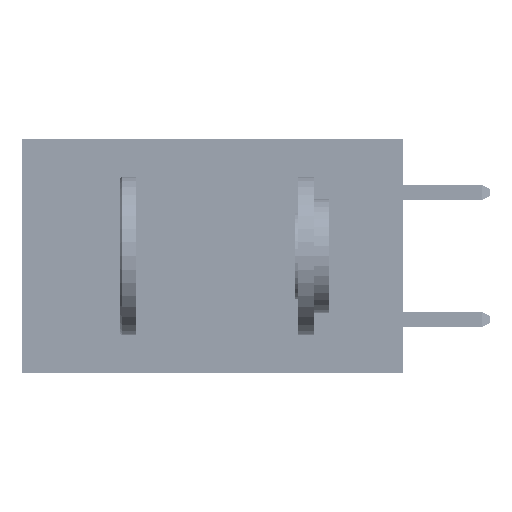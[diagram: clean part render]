
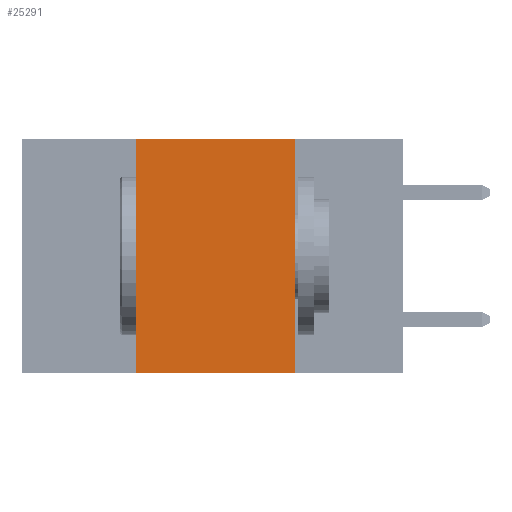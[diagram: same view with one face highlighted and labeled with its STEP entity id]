
A CAD part, left-side view. The second image highlights one B-rep face of the part: STEP entity #25291.
In plain terms, the highlighted planar face has unit normal (-1, 0, 0).
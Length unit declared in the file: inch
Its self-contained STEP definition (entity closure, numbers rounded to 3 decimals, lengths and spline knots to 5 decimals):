
#293 = DIRECTION ( 'NONE',  ( 0., -1., 0. ) ) ;
#961 = EDGE_CURVE ( 'NONE', #30247, #11524, #12886, .T. ) ;
#1838 = DIRECTION ( 'NONE',  ( 0., -1., 0. ) ) ;
#3914 = LINE ( 'NONE', #35413, #33627 ) ;
#4728 = EDGE_CURVE ( 'NONE', #30854, #30247, #3914, .T. ) ;
#6305 = FACE_OUTER_BOUND ( 'NONE', #22208, .T. ) ;
#8317 = DIRECTION ( 'NONE',  ( 0., 0., 1. ) ) ;
#9486 = CARTESIAN_POINT ( 'NONE',  ( 0., 0.17, 0. ) ) ;
#10294 = ORIENTED_EDGE ( 'NONE', *, *, #961, .F. ) ;
#10881 = CARTESIAN_POINT ( 'NONE',  ( 0., 0.42, -0.37 ) ) ;
#11524 = VERTEX_POINT ( 'NONE', #44864 ) ;
#12886 = LINE ( 'NONE', #13642, #32213 ) ;
#13642 = CARTESIAN_POINT ( 'NONE',  ( 0., 0.6, 0. ) ) ;
#14005 = VERTEX_POINT ( 'NONE', #34149 ) ;
#18657 = PLANE ( 'NONE',  #36313 ) ;
#22208 = EDGE_LOOP ( 'NONE', ( #46524, #10294, #30908, #36912 ) ) ;
#22333 = VECTOR ( 'NONE', #32714, 39.37008 ) ;
#22522 = DIRECTION ( 'NONE',  ( 1., 0., 0. ) ) ;
#25291 = ADVANCED_FACE ( 'NONE', ( #6305 ), #18657, .F. ) ;
#27451 = CARTESIAN_POINT ( 'NONE',  ( 0., 0.6, -0.37 ) ) ;
#28456 = EDGE_CURVE ( 'NONE', #30854, #14005, #45383, .T. ) ;
#30247 = VERTEX_POINT ( 'NONE', #45873 ) ;
#30854 = VERTEX_POINT ( 'NONE', #10881 ) ;
#30908 = ORIENTED_EDGE ( 'NONE', *, *, #4728, .F. ) ;
#32213 = VECTOR ( 'NONE', #1838, 39.37008 ) ;
#32574 = LINE ( 'NONE', #9486, #22333 ) ;
#32714 = DIRECTION ( 'NONE',  ( 0., 0., -1. ) ) ;
#33627 = VECTOR ( 'NONE', #8317, 39.37008 ) ;
#34149 = CARTESIAN_POINT ( 'NONE',  ( 0., 0.17, -0.37 ) ) ;
#34664 = EDGE_CURVE ( 'NONE', #11524, #14005, #32574, .T. ) ;
#35413 = CARTESIAN_POINT ( 'NONE',  ( 0., 0.42, 0. ) ) ;
#36313 = AXIS2_PLACEMENT_3D ( 'NONE', #41677, #22522, #49398 ) ;
#36912 = ORIENTED_EDGE ( 'NONE', *, *, #28456, .T. ) ;
#41677 = CARTESIAN_POINT ( 'NONE',  ( 0., 0.6, 0. ) ) ;
#42966 = VECTOR ( 'NONE', #293, 39.37008 ) ;
#44864 = CARTESIAN_POINT ( 'NONE',  ( 0., 0.17, 0. ) ) ;
#45383 = LINE ( 'NONE', #27451, #42966 ) ;
#45873 = CARTESIAN_POINT ( 'NONE',  ( 0., 0.42, 0. ) ) ;
#46524 = ORIENTED_EDGE ( 'NONE', *, *, #34664, .F. ) ;
#49398 = DIRECTION ( 'NONE',  ( 0., 0., -1. ) ) ;
